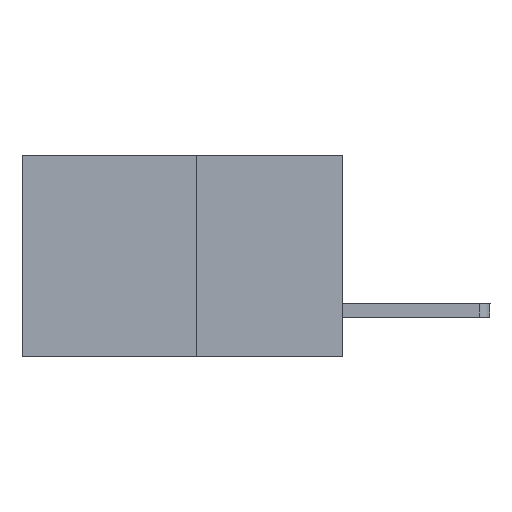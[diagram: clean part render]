
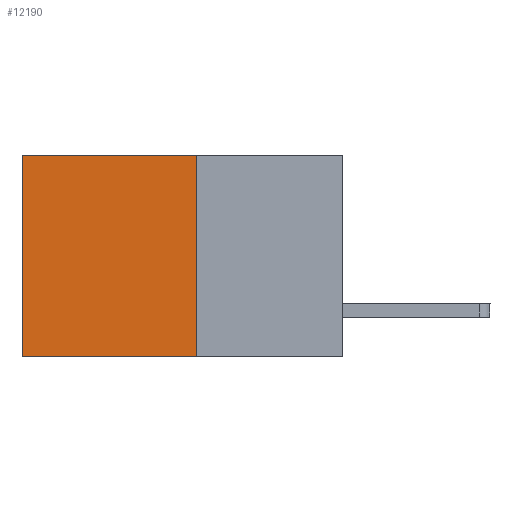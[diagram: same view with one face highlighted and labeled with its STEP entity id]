
A CAD part, left-side view. The second image highlights one B-rep face of the part: STEP entity #12190.
In plain terms, the highlighted planar face has unit normal (-1, 0, 0).
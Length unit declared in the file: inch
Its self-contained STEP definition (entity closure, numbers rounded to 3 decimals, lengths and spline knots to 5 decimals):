
#745 = VECTOR ( 'NONE', #6847, 39.37008 ) ;
#1574 = VERTEX_POINT ( 'NONE', #3596 ) ;
#1615 = ORIENTED_EDGE ( 'NONE', *, *, #5643, .T. ) ;
#1808 = ORIENTED_EDGE ( 'NONE', *, *, #8311, .T. ) ;
#1852 = ORIENTED_EDGE ( 'NONE', *, *, #10653, .F. ) ;
#2121 = DIRECTION ( 'NONE',  ( 0., 0., -1. ) ) ;
#2285 = CARTESIAN_POINT ( 'NONE',  ( 0.277, 0.27, 0. ) ) ;
#3002 = CARTESIAN_POINT ( 'NONE',  ( 0.277, 0.27, -0.37 ) ) ;
#3484 = CARTESIAN_POINT ( 'NONE',  ( 0.277, 0.27, -0.37 ) ) ;
#3596 = CARTESIAN_POINT ( 'NONE',  ( 0.277, 0.59, -0.37 ) ) ;
#3845 = LINE ( 'NONE', #4945, #5802 ) ;
#4091 = EDGE_LOOP ( 'NONE', ( #1808, #1852, #10706, #1615 ) ) ;
#4092 = CARTESIAN_POINT ( 'NONE',  ( 0.277, 0.27, -0.37 ) ) ;
#4460 = AXIS2_PLACEMENT_3D ( 'NONE', #4092, #7983, #2121 ) ;
#4945 = CARTESIAN_POINT ( 'NONE',  ( 0.277, 0.59, -0.37 ) ) ;
#5643 = EDGE_CURVE ( 'NONE', #8543, #8467, #10609, .T. ) ;
#5704 = CARTESIAN_POINT ( 'NONE',  ( 0.277, 0.27, 0. ) ) ;
#5802 = VECTOR ( 'NONE', #10682, 39.37008 ) ;
#6067 = LINE ( 'NONE', #3002, #745 ) ;
#6390 = LINE ( 'NONE', #11377, #11248 ) ;
#6550 = DIRECTION ( 'NONE',  ( 0., 0., -1. ) ) ;
#6847 = DIRECTION ( 'NONE',  ( 0., 1., 0. ) ) ;
#7561 = FACE_OUTER_BOUND ( 'NONE', #4091, .T. ) ;
#7742 = VECTOR ( 'NONE', #10069, 39.37008 ) ;
#7983 = DIRECTION ( 'NONE',  ( 1., 0., 0. ) ) ;
#8311 = EDGE_CURVE ( 'NONE', #8467, #1574, #3845, .T. ) ;
#8467 = VERTEX_POINT ( 'NONE', #9410 ) ;
#8543 = VERTEX_POINT ( 'NONE', #5704 ) ;
#9074 = EDGE_CURVE ( 'NONE', #8543, #12384, #6390, .T. ) ;
#9410 = CARTESIAN_POINT ( 'NONE',  ( 0.277, 0.59, 0. ) ) ;
#10069 = DIRECTION ( 'NONE',  ( 0., 1., 0. ) ) ;
#10609 = LINE ( 'NONE', #2285, #7742 ) ;
#10653 = EDGE_CURVE ( 'NONE', #12384, #1574, #6067, .T. ) ;
#10682 = DIRECTION ( 'NONE',  ( 0., 0., -1. ) ) ;
#10706 = ORIENTED_EDGE ( 'NONE', *, *, #9074, .F. ) ;
#10859 = PLANE ( 'NONE',  #4460 ) ;
#11248 = VECTOR ( 'NONE', #6550, 39.37008 ) ;
#11377 = CARTESIAN_POINT ( 'NONE',  ( 0.277, 0.27, -0.37 ) ) ;
#12190 = ADVANCED_FACE ( 'NONE', ( #7561 ), #10859, .F. ) ;
#12384 = VERTEX_POINT ( 'NONE', #3484 ) ;
